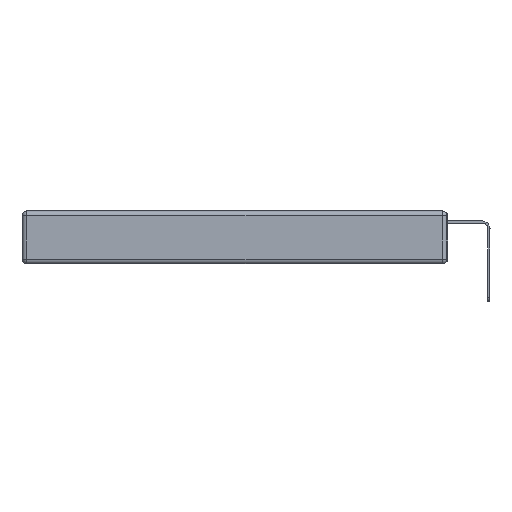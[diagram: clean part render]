
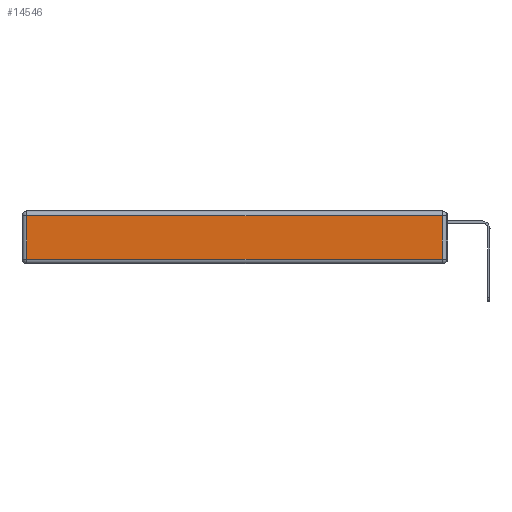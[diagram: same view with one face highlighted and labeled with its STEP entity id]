
A CAD part, left-side view. The second image highlights one B-rep face of the part: STEP entity #14546.
In plain terms, the highlighted planar face has unit normal (-1, 0, 0).
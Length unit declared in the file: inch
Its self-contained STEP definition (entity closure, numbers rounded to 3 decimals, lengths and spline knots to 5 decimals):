
#220 = ORIENTED_EDGE ( 'NONE', *, *, #1133, .T. ) ;
#377 = VERTEX_POINT ( 'NONE', #18752 ) ;
#1133 = EDGE_CURVE ( 'NONE', #3516, #23416, #4698, .T. ) ;
#2193 = CARTESIAN_POINT ( 'NONE',  ( 0., 2.72, -0.03 ) ) ;
#2914 = EDGE_CURVE ( 'NONE', #5476, #377, #4862, .T. ) ;
#3171 = EDGE_LOOP ( 'NONE', ( #12129, #23281, #220, #9790 ) ) ;
#3516 = VERTEX_POINT ( 'NONE', #22282 ) ;
#4158 = LINE ( 'NONE', #10426, #16396 ) ;
#4698 = LINE ( 'NONE', #7348, #17508 ) ;
#4862 = LINE ( 'NONE', #13223, #14544 ) ;
#5476 = VERTEX_POINT ( 'NONE', #11746 ) ;
#6261 = CARTESIAN_POINT ( 'NONE',  ( 0., 0., -0.343 ) ) ;
#6265 = EDGE_CURVE ( 'NONE', #23416, #5476, #15524, .T. ) ;
#7348 = CARTESIAN_POINT ( 'NONE',  ( 0., 2.75, -0.03 ) ) ;
#7876 = DIRECTION ( 'NONE',  ( 0., -1., 0. ) ) ;
#9654 = FACE_OUTER_BOUND ( 'NONE', #3171, .T. ) ;
#9790 = ORIENTED_EDGE ( 'NONE', *, *, #6265, .T. ) ;
#10426 = CARTESIAN_POINT ( 'NONE',  ( 0., 0.03, -0.343 ) ) ;
#11746 = CARTESIAN_POINT ( 'NONE',  ( 0., 2.72, -0.313 ) ) ;
#11813 = VECTOR ( 'NONE', #13954, 39.37008 ) ;
#11914 = PLANE ( 'NONE',  #15237 ) ;
#12129 = ORIENTED_EDGE ( 'NONE', *, *, #2914, .T. ) ;
#13223 = CARTESIAN_POINT ( 'NONE',  ( 0., 0., -0.313 ) ) ;
#13954 = DIRECTION ( 'NONE',  ( 0., 0., -1. ) ) ;
#14304 = DIRECTION ( 'NONE',  ( 0., 0., 1. ) ) ;
#14441 = DIRECTION ( 'NONE',  ( 0., 1., 0. ) ) ;
#14544 = VECTOR ( 'NONE', #7876, 39.37008 ) ;
#14546 = ADVANCED_FACE ( 'NONE', ( #9654 ), #11914, .T. ) ;
#15237 = AXIS2_PLACEMENT_3D ( 'NONE', #6261, #19285, #15431 ) ;
#15431 = DIRECTION ( 'NONE',  ( 0., 0., 1. ) ) ;
#15524 = LINE ( 'NONE', #19264, #11813 ) ;
#16396 = VECTOR ( 'NONE', #14304, 39.37008 ) ;
#16594 = EDGE_CURVE ( 'NONE', #377, #3516, #4158, .T. ) ;
#17508 = VECTOR ( 'NONE', #14441, 39.37008 ) ;
#18752 = CARTESIAN_POINT ( 'NONE',  ( 0., 0.03, -0.313 ) ) ;
#19264 = CARTESIAN_POINT ( 'NONE',  ( 0., 2.72, -0.343 ) ) ;
#19285 = DIRECTION ( 'NONE',  ( -1., 0., 0. ) ) ;
#22282 = CARTESIAN_POINT ( 'NONE',  ( 0., 0.03, -0.03 ) ) ;
#23281 = ORIENTED_EDGE ( 'NONE', *, *, #16594, .T. ) ;
#23416 = VERTEX_POINT ( 'NONE', #2193 ) ;
